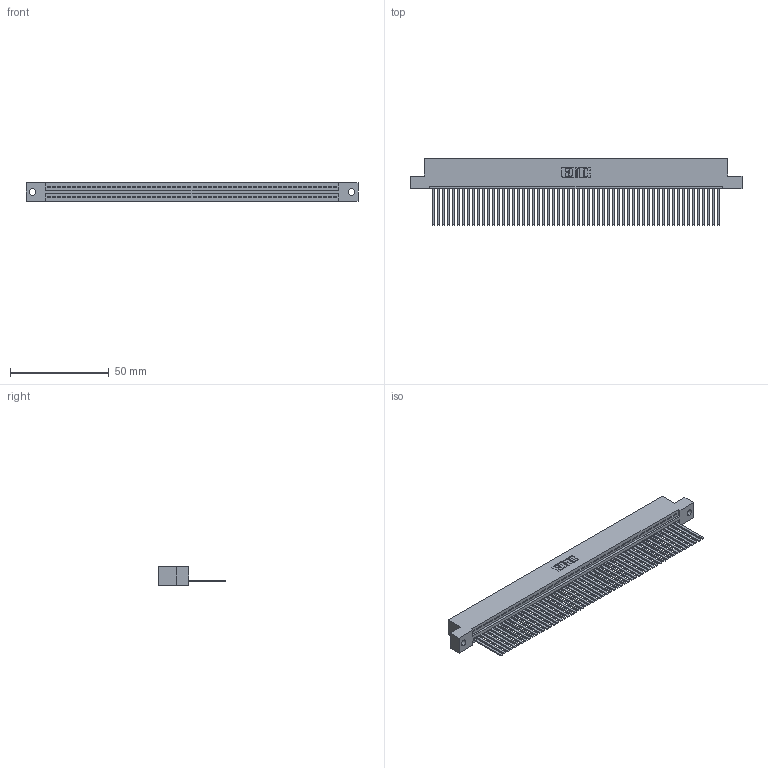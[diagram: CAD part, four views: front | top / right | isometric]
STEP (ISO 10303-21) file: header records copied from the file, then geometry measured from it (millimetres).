
FILE_DESCRIPTION (( 'STEP AP203' ), '1' );
FILE_NAME ('345-058-544-102.STEP', '2018-09-26T15:46:11', ( '' ), ( '' ), 'SwSTEP 2.0', 'SolidWorks 2016', '' );
FILE_SCHEMA (( 'CONFIG_CONTROL_DESIGN' ));
Length unit declared in the file: inch
Products named in the file (3): 345 Part_Flush Mounting Lugs - 0.128 Dia; 345-292-001_345-293-144; 345-058-544-102
Assembly tree (59 placements, depth 2):
  345-058-544-102
    345 Part_Flush Mounting Lugs - 0.128 Dia
    345-292-001_345-293-144  x58
Bounding box: 168.53 x 33.96 x 9.4 mm (x, y, z)
Volume: 16773.1 mm3; surface area: 24252.5 mm2
Topology: 59 solids, 59 shells, 3142 faces, 9505 edges, 6258 vertices
Faces by surface type: plane 2168, cylinder 974
Entity records: 41317 total; most frequent: CARTESIAN_POINT 7162, ORIENTED_EDGE 7154, DIRECTION 6229, EDGE_CURVE 3577, VECTOR 3217, LINE 3217, VERTEX_POINT 2382, AXIS2_PLACEMENT_3D 1506
